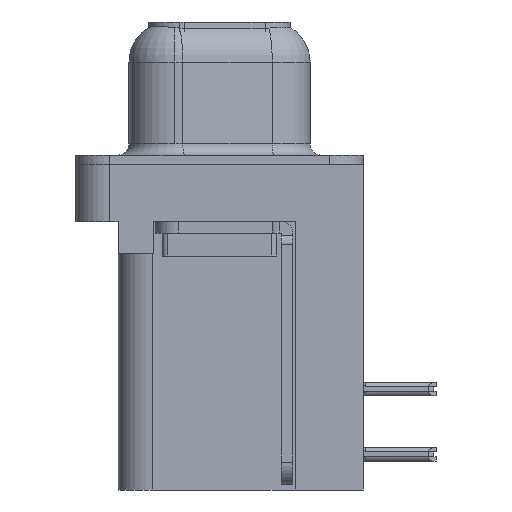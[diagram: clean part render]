
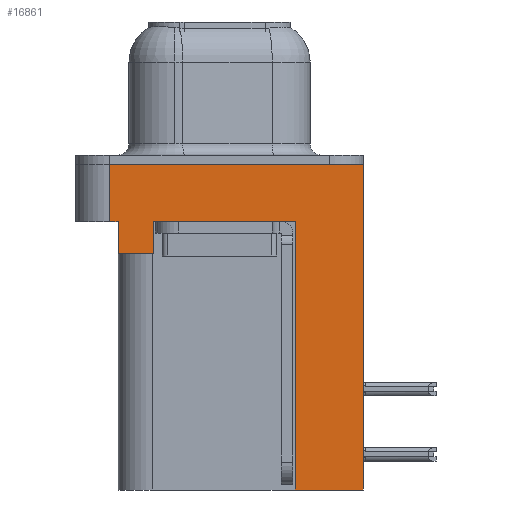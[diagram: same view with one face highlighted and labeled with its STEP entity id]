
A CAD part, left-side view. The second image highlights one B-rep face of the part: STEP entity #16861.
In plain terms, the highlighted planar face has unit normal (-1, 0, 0).
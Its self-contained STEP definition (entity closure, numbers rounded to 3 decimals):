
#103 = VERTEX_POINT ( 'NONE', #24323 ) ;
#1253 = VERTEX_POINT ( 'NONE', #5525 ) ;
#1341 = ORIENTED_EDGE ( 'NONE', *, *, #19353, .F. ) ;
#1453 = ORIENTED_EDGE ( 'NONE', *, *, #2893, .T. ) ;
#1454 = ORIENTED_EDGE ( 'NONE', *, *, #27212, .T. ) ;
#1702 = VERTEX_POINT ( 'NONE', #1997 ) ;
#1997 = CARTESIAN_POINT ( 'NONE',  ( -3., -6.275, 0. ) ) ;
#2413 = DIRECTION ( 'NONE',  ( 0., 0., 1. ) ) ;
#2874 = EDGE_CURVE ( 'NONE', #13803, #9202, #24904, .T. ) ;
#2893 = EDGE_CURVE ( 'NONE', #17345, #1253, #20118, .T. ) ;
#3005 = ORIENTED_EDGE ( 'NONE', *, *, #2874, .F. ) ;
#3145 = LINE ( 'NONE', #11960, #17729 ) ;
#3849 = EDGE_CURVE ( 'NONE', #21577, #1702, #8324, .T. ) ;
#4145 = CARTESIAN_POINT ( 'NONE',  ( -3., 4.775, -2.5 ) ) ;
#4262 = CARTESIAN_POINT ( 'NONE',  ( -3., 2.895, -3.9 ) ) ;
#4309 = CARTESIAN_POINT ( 'NONE',  ( -3., 4.775, -2.5 ) ) ;
#4828 = ORIENTED_EDGE ( 'NONE', *, *, #7707, .F. ) ;
#5019 = DIRECTION ( 'NONE',  ( 0., 0., 1. ) ) ;
#5525 = CARTESIAN_POINT ( 'NONE',  ( -3., 2.895, -2.5 ) ) ;
#6245 = CARTESIAN_POINT ( 'NONE',  ( -3., -3.295, -2.5 ) ) ;
#6470 = CARTESIAN_POINT ( 'NONE',  ( -3., -6.275, 0. ) ) ;
#6612 = DIRECTION ( 'NONE',  ( -1., 0., 0. ) ) ;
#7690 = EDGE_CURVE ( 'NONE', #12248, #28248, #26090, .T. ) ;
#7707 = EDGE_CURVE ( 'NONE', #28248, #1702, #17478, .T. ) ;
#7857 = VECTOR ( 'NONE', #24656, 1000. ) ;
#8182 = EDGE_LOOP ( 'NONE', ( #4828, #13805, #1454, #3005, #12337, #1453, #14702, #1341, #9790, #22116 ) ) ;
#8324 = LINE ( 'NONE', #17166, #11859 ) ;
#9202 = VERTEX_POINT ( 'NONE', #10788 ) ;
#9210 = DIRECTION ( 'NONE',  ( 0., 0., 1. ) ) ;
#9481 = LINE ( 'NONE', #16142, #18190 ) ;
#9790 = ORIENTED_EDGE ( 'NONE', *, *, #22790, .F. ) ;
#10788 = CARTESIAN_POINT ( 'NONE',  ( -3., 4.425, -2.5 ) ) ;
#10911 = VECTOR ( 'NONE', #28539, 1000. ) ;
#11093 = CARTESIAN_POINT ( 'NONE',  ( -3., -6.275, -2.5 ) ) ;
#11531 = CARTESIAN_POINT ( 'NONE',  ( -3., 4.425, -3.9 ) ) ;
#11859 = VECTOR ( 'NONE', #26340, 1000. ) ;
#11960 = CARTESIAN_POINT ( 'NONE',  ( -3., -6.275, -2.5 ) ) ;
#12248 = VERTEX_POINT ( 'NONE', #4145 ) ;
#12337 = ORIENTED_EDGE ( 'NONE', *, *, #21065, .F. ) ;
#13038 = VERTEX_POINT ( 'NONE', #6245 ) ;
#13803 = VERTEX_POINT ( 'NONE', #18268 ) ;
#13805 = ORIENTED_EDGE ( 'NONE', *, *, #7690, .F. ) ;
#13829 = AXIS2_PLACEMENT_3D ( 'NONE', #11093, #6612, #2413 ) ;
#14702 = ORIENTED_EDGE ( 'NONE', *, *, #25118, .T. ) ;
#14895 = VECTOR ( 'NONE', #15308, 1000. ) ;
#15308 = DIRECTION ( 'NONE',  ( 0., -1., 0. ) ) ;
#16142 = CARTESIAN_POINT ( 'NONE',  ( -3., -3.295, -14.2 ) ) ;
#16161 = DIRECTION ( 'NONE',  ( 0., -1., 0. ) ) ;
#16200 = CARTESIAN_POINT ( 'NONE',  ( -3., -3.295, -14.2 ) ) ;
#16356 = LINE ( 'NONE', #16200, #7857 ) ;
#16861 = ADVANCED_FACE ( 'NONE', ( #21854 ), #20104, .T. ) ;
#17166 = CARTESIAN_POINT ( 'NONE',  ( -3., -6.275, -2.5 ) ) ;
#17175 = VECTOR ( 'NONE', #27233, 1000. ) ;
#17292 = CARTESIAN_POINT ( 'NONE',  ( -3., 4.775, 0. ) ) ;
#17345 = VERTEX_POINT ( 'NONE', #4262 ) ;
#17478 = LINE ( 'NONE', #6470, #14895 ) ;
#17600 = VECTOR ( 'NONE', #27478, 1000. ) ;
#17729 = VECTOR ( 'NONE', #16161, 1000. ) ;
#18190 = VECTOR ( 'NONE', #27076, 1000. ) ;
#18268 = CARTESIAN_POINT ( 'NONE',  ( -3., 4.425, -3.9 ) ) ;
#19353 = EDGE_CURVE ( 'NONE', #103, #13038, #16356, .T. ) ;
#20104 = PLANE ( 'NONE',  #13829 ) ;
#20118 = LINE ( 'NONE', #27096, #24393 ) ;
#20190 = CARTESIAN_POINT ( 'NONE',  ( -3., -6.275, -2.5 ) ) ;
#20547 = CARTESIAN_POINT ( 'NONE',  ( -3., 4.425, -3.9 ) ) ;
#20613 = VECTOR ( 'NONE', #9210, 1000. ) ;
#21065 = EDGE_CURVE ( 'NONE', #17345, #13803, #25216, .T. ) ;
#21577 = VERTEX_POINT ( 'NONE', #23876 ) ;
#21854 = FACE_OUTER_BOUND ( 'NONE', #8182, .T. ) ;
#22116 = ORIENTED_EDGE ( 'NONE', *, *, #3849, .T. ) ;
#22387 = LINE ( 'NONE', #20190, #17600 ) ;
#22790 = EDGE_CURVE ( 'NONE', #21577, #103, #9481, .T. ) ;
#23876 = CARTESIAN_POINT ( 'NONE',  ( -3., -6.275, -14.2 ) ) ;
#24323 = CARTESIAN_POINT ( 'NONE',  ( -3., -3.295, -14.2 ) ) ;
#24393 = VECTOR ( 'NONE', #5019, 1000. ) ;
#24656 = DIRECTION ( 'NONE',  ( 0., 0., 1. ) ) ;
#24904 = LINE ( 'NONE', #20547, #20613 ) ;
#25118 = EDGE_CURVE ( 'NONE', #1253, #13038, #3145, .T. ) ;
#25216 = LINE ( 'NONE', #11531, #17175 ) ;
#26090 = LINE ( 'NONE', #4309, #10911 ) ;
#26340 = DIRECTION ( 'NONE',  ( 0., 0., 1. ) ) ;
#27076 = DIRECTION ( 'NONE',  ( 0., 1., 0. ) ) ;
#27096 = CARTESIAN_POINT ( 'NONE',  ( -3., 2.895, -3.9 ) ) ;
#27212 = EDGE_CURVE ( 'NONE', #12248, #9202, #22387, .T. ) ;
#27233 = DIRECTION ( 'NONE',  ( 0., 1., 0. ) ) ;
#27478 = DIRECTION ( 'NONE',  ( 0., -1., 0. ) ) ;
#28248 = VERTEX_POINT ( 'NONE', #17292 ) ;
#28539 = DIRECTION ( 'NONE',  ( 0., 0., 1. ) ) ;
